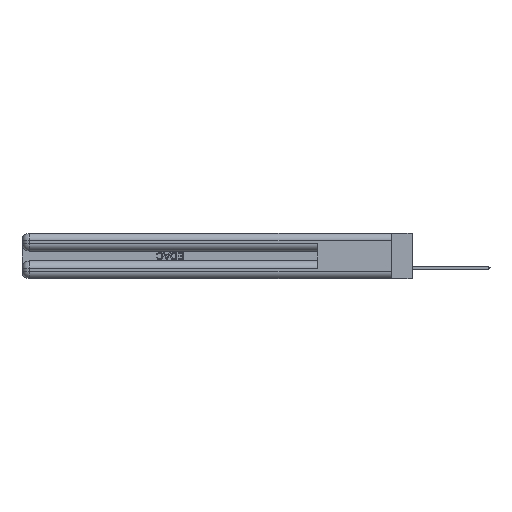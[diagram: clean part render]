
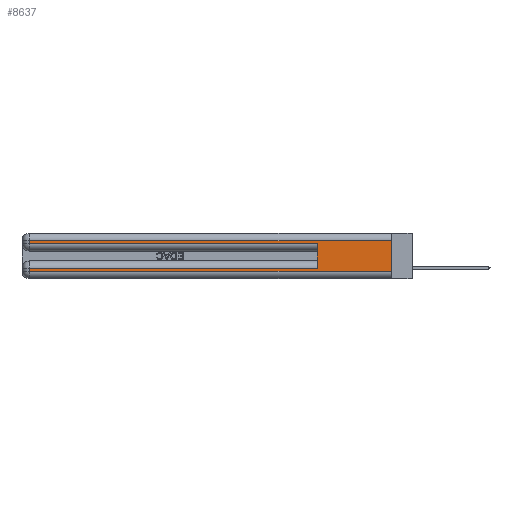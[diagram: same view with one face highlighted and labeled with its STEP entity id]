
A CAD part, left-side view. The second image highlights one B-rep face of the part: STEP entity #8637.
In plain terms, the highlighted planar face has unit normal (-1, 0, 0).
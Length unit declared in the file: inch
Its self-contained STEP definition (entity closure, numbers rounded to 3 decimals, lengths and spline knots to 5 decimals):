
#512 = EDGE_CURVE ( 'NONE', #31478, #2074, #13204, .T. ) ;
#543 = VECTOR ( 'NONE', #1982, 39.37008 ) ;
#1081 = DIRECTION ( 'NONE',  ( 0., 1., 0. ) ) ;
#1877 = VECTOR ( 'NONE', #5812, 39.37008 ) ;
#1982 = DIRECTION ( 'NONE',  ( 0., -1., 0. ) ) ;
#2037 = ORIENTED_EDGE ( 'NONE', *, *, #5425, .T. ) ;
#2074 = VERTEX_POINT ( 'NONE', #7553 ) ;
#2188 = VERTEX_POINT ( 'NONE', #15969 ) ;
#3173 = DIRECTION ( 'NONE',  ( 0., 0., -1. ) ) ;
#3893 = EDGE_CURVE ( 'NONE', #4384, #2188, #18636, .T. ) ;
#4384 = VERTEX_POINT ( 'NONE', #32827 ) ;
#4529 = ORIENTED_EDGE ( 'NONE', *, *, #27355, .F. ) ;
#5425 = EDGE_CURVE ( 'NONE', #17385, #36523, #14016, .T. ) ;
#5812 = DIRECTION ( 'NONE',  ( 0., 1., 0. ) ) ;
#6922 = CARTESIAN_POINT ( 'NONE',  ( 0., 0., 0.37 ) ) ;
#7207 = PLANE ( 'NONE',  #15358 ) ;
#7553 = CARTESIAN_POINT ( 'NONE',  ( 0., 2.94, 0.31 ) ) ;
#7978 = CARTESIAN_POINT ( 'NONE',  ( 0., 0.6, 0.145 ) ) ;
#8150 = DIRECTION ( 'NONE',  ( 0., 0., 1. ) ) ;
#8637 = ADVANCED_FACE ( 'NONE', ( #45370 ), #7207, .F. ) ;
#8753 = VECTOR ( 'NONE', #1081, 39.37008 ) ;
#9524 = LINE ( 'NONE', #22537, #543 ) ;
#9607 = CARTESIAN_POINT ( 'NONE',  ( 0., 0., 0.06 ) ) ;
#10583 = ORIENTED_EDGE ( 'NONE', *, *, #19576, .T. ) ;
#11256 = CARTESIAN_POINT ( 'NONE',  ( 0., 0.6, 0.085 ) ) ;
#13204 = LINE ( 'NONE', #29350, #8753 ) ;
#13384 = EDGE_CURVE ( 'NONE', #2074, #4384, #18887, .T. ) ;
#14016 = LINE ( 'NONE', #26374, #1877 ) ;
#15358 = AXIS2_PLACEMENT_3D ( 'NONE', #35813, #23638, #45456 ) ;
#15749 = VECTOR ( 'NONE', #41491, 39.37008 ) ;
#15888 = DIRECTION ( 'NONE',  ( 0., -1., 0. ) ) ;
#15969 = CARTESIAN_POINT ( 'NONE',  ( 0., 0.6, 0.285 ) ) ;
#16492 = ORIENTED_EDGE ( 'NONE', *, *, #22795, .F. ) ;
#16941 = CARTESIAN_POINT ( 'NONE',  ( 0., 0., 0.31 ) ) ;
#17036 = EDGE_LOOP ( 'NONE', ( #16492, #40417, #47294, #39818, #4529, #2037, #27271, #10583 ) ) ;
#17385 = VERTEX_POINT ( 'NONE', #11256 ) ;
#18636 = LINE ( 'NONE', #40397, #33975 ) ;
#18887 = LINE ( 'NONE', #52903, #15749 ) ;
#19576 = EDGE_CURVE ( 'NONE', #35876, #28185, #9524, .T. ) ;
#22537 = CARTESIAN_POINT ( 'NONE',  ( 0., 0., 0.06 ) ) ;
#22795 = EDGE_CURVE ( 'NONE', #31478, #28185, #31731, .T. ) ;
#23638 = DIRECTION ( 'NONE',  ( 1., 0., 0. ) ) ;
#26374 = CARTESIAN_POINT ( 'NONE',  ( 0., 0., 0.085 ) ) ;
#27271 = ORIENTED_EDGE ( 'NONE', *, *, #29615, .T. ) ;
#27355 = EDGE_CURVE ( 'NONE', #17385, #2188, #45114, .T. ) ;
#27385 = DIRECTION ( 'NONE',  ( 0., 0., -1. ) ) ;
#28185 = VERTEX_POINT ( 'NONE', #9607 ) ;
#28518 = VECTOR ( 'NONE', #8150, 39.37008 ) ;
#29350 = CARTESIAN_POINT ( 'NONE',  ( 0., 0., 0.31 ) ) ;
#29615 = EDGE_CURVE ( 'NONE', #36523, #35876, #45531, .T. ) ;
#31478 = VERTEX_POINT ( 'NONE', #16941 ) ;
#31731 = LINE ( 'NONE', #6922, #32969 ) ;
#32827 = CARTESIAN_POINT ( 'NONE',  ( 0., 2.94, 0.285 ) ) ;
#32969 = VECTOR ( 'NONE', #3173, 39.37008 ) ;
#33975 = VECTOR ( 'NONE', #15888, 39.37008 ) ;
#35813 = CARTESIAN_POINT ( 'NONE',  ( 0., 0., 0.37 ) ) ;
#35876 = VERTEX_POINT ( 'NONE', #43246 ) ;
#36523 = VERTEX_POINT ( 'NONE', #49592 ) ;
#39818 = ORIENTED_EDGE ( 'NONE', *, *, #3893, .T. ) ;
#40397 = CARTESIAN_POINT ( 'NONE',  ( 0., 0., 0.285 ) ) ;
#40417 = ORIENTED_EDGE ( 'NONE', *, *, #512, .T. ) ;
#41491 = DIRECTION ( 'NONE',  ( 0., 0., -1. ) ) ;
#43246 = CARTESIAN_POINT ( 'NONE',  ( 0., 2.94, 0.06 ) ) ;
#44342 = VECTOR ( 'NONE', #27385, 39.37008 ) ;
#45114 = LINE ( 'NONE', #7978, #28518 ) ;
#45370 = FACE_OUTER_BOUND ( 'NONE', #17036, .T. ) ;
#45456 = DIRECTION ( 'NONE',  ( 0., 0., -1. ) ) ;
#45531 = LINE ( 'NONE', #49520, #44342 ) ;
#47294 = ORIENTED_EDGE ( 'NONE', *, *, #13384, .T. ) ;
#49520 = CARTESIAN_POINT ( 'NONE',  ( 0., 2.94, 0.37 ) ) ;
#49592 = CARTESIAN_POINT ( 'NONE',  ( 0., 2.94, 0.085 ) ) ;
#52903 = CARTESIAN_POINT ( 'NONE',  ( 0., 2.94, 0.37 ) ) ;
